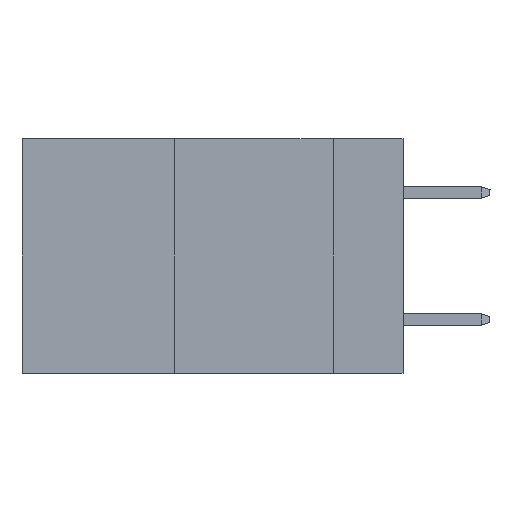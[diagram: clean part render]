
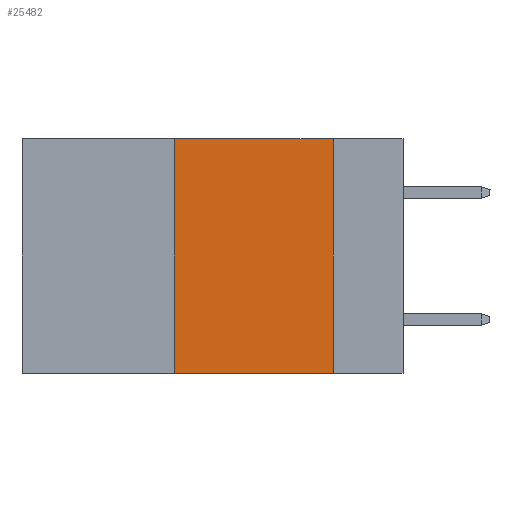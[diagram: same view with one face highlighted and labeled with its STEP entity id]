
A CAD part, left-side view. The second image highlights one B-rep face of the part: STEP entity #25482.
In plain terms, the highlighted planar face has unit normal (-1, 0, 0).
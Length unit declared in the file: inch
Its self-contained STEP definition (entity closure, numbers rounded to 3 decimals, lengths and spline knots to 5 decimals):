
#1584 = EDGE_CURVE ( 'NONE', #4344, #11949, #17836, .T. ) ;
#2341 = AXIS2_PLACEMENT_3D ( 'NONE', #20274, #14035, #25031 ) ;
#2645 = PLANE ( 'NONE',  #2341 ) ;
#3730 = VERTEX_POINT ( 'NONE', #5598 ) ;
#4344 = VERTEX_POINT ( 'NONE', #23774 ) ;
#5260 = ORIENTED_EDGE ( 'NONE', *, *, #25550, .F. ) ;
#5598 = CARTESIAN_POINT ( 'NONE',  ( 0., 0.11, -0.37 ) ) ;
#6219 = CARTESIAN_POINT ( 'NONE',  ( 0., 0.36, -0.37 ) ) ;
#6847 = CARTESIAN_POINT ( 'NONE',  ( 0., 0.6, 0. ) ) ;
#7376 = DIRECTION ( 'NONE',  ( 0., -1., 0. ) ) ;
#8315 = VECTOR ( 'NONE', #27344, 39.37008 ) ;
#10616 = ORIENTED_EDGE ( 'NONE', *, *, #24785, .T. ) ;
#10716 = EDGE_CURVE ( 'NONE', #11949, #3730, #27627, .T. ) ;
#11949 = VERTEX_POINT ( 'NONE', #18848 ) ;
#14035 = DIRECTION ( 'NONE',  ( 1., 0., 0. ) ) ;
#14163 = CARTESIAN_POINT ( 'NONE',  ( 0., 0.11, 0. ) ) ;
#16289 = CARTESIAN_POINT ( 'NONE',  ( 0., 0.6, -0.37 ) ) ;
#17540 = VECTOR ( 'NONE', #25105, 39.37008 ) ;
#17836 = LINE ( 'NONE', #6847, #18063 ) ;
#18063 = VECTOR ( 'NONE', #7376, 39.37008 ) ;
#18093 = ORIENTED_EDGE ( 'NONE', *, *, #10716, .F. ) ;
#18394 = FACE_OUTER_BOUND ( 'NONE', #23410, .T. ) ;
#18848 = CARTESIAN_POINT ( 'NONE',  ( 0., 0.11, 0. ) ) ;
#19119 = DIRECTION ( 'NONE',  ( 0., 0., -1. ) ) ;
#20274 = CARTESIAN_POINT ( 'NONE',  ( 0., 0.6, 0. ) ) ;
#21366 = ORIENTED_EDGE ( 'NONE', *, *, #1584, .F. ) ;
#22723 = CARTESIAN_POINT ( 'NONE',  ( 0., 0.36, 0. ) ) ;
#23410 = EDGE_LOOP ( 'NONE', ( #18093, #21366, #5260, #10616 ) ) ;
#23774 = CARTESIAN_POINT ( 'NONE',  ( 0., 0.36, 0. ) ) ;
#24785 = EDGE_CURVE ( 'NONE', #26780, #3730, #25535, .T. ) ;
#24883 = LINE ( 'NONE', #22723, #8315 ) ;
#25007 = VECTOR ( 'NONE', #19119, 39.37008 ) ;
#25031 = DIRECTION ( 'NONE',  ( 0., 0., -1. ) ) ;
#25105 = DIRECTION ( 'NONE',  ( 0., -1., 0. ) ) ;
#25482 = ADVANCED_FACE ( 'NONE', ( #18394 ), #2645, .F. ) ;
#25535 = LINE ( 'NONE', #16289, #17540 ) ;
#25550 = EDGE_CURVE ( 'NONE', #26780, #4344, #24883, .T. ) ;
#26780 = VERTEX_POINT ( 'NONE', #6219 ) ;
#27344 = DIRECTION ( 'NONE',  ( 0., 0., 1. ) ) ;
#27627 = LINE ( 'NONE', #14163, #25007 ) ;
